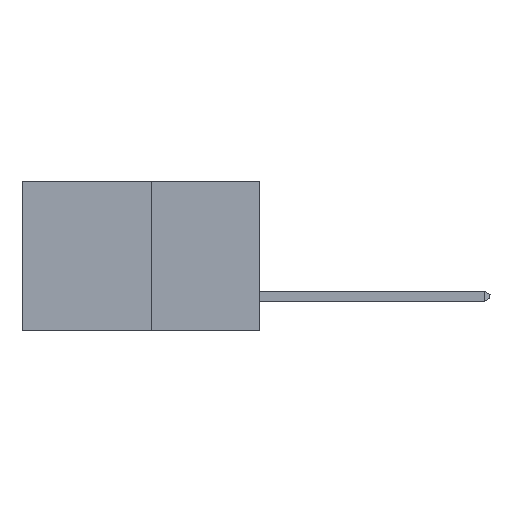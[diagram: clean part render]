
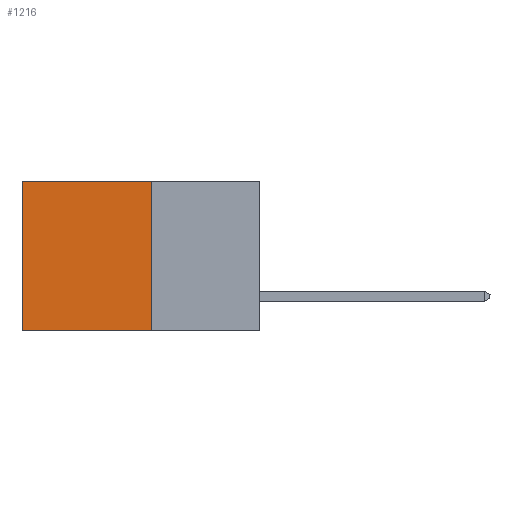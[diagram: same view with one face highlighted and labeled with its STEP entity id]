
A CAD part, left-side view. The second image highlights one B-rep face of the part: STEP entity #1216.
In plain terms, the highlighted planar face has unit normal (-1, 0, 0).
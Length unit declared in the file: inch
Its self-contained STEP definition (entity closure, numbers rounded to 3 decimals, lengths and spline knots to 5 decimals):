
#424 = CARTESIAN_POINT ( 'NONE',  ( 0.277, 0.27, -0.37 ) ) ;
#1216 = ADVANCED_FACE ( 'NONE', ( #18687 ), #19611, .F. ) ;
#1347 = EDGE_CURVE ( 'NONE', #5961, #11476, #3356, .T. ) ;
#3080 = VERTEX_POINT ( 'NONE', #15899 ) ;
#3356 = LINE ( 'NONE', #9914, #12105 ) ;
#3727 = VECTOR ( 'NONE', #16318, 39.37008 ) ;
#4156 = CARTESIAN_POINT ( 'NONE',  ( 0.277, 0.59, -0.37 ) ) ;
#4184 = CARTESIAN_POINT ( 'NONE',  ( 0.277, 0.27, 0. ) ) ;
#4206 = LINE ( 'NONE', #10052, #21698 ) ;
#4679 = LINE ( 'NONE', #14429, #18317 ) ;
#5961 = VERTEX_POINT ( 'NONE', #4184 ) ;
#8259 = ORIENTED_EDGE ( 'NONE', *, *, #1347, .F. ) ;
#9725 = DIRECTION ( 'NONE',  ( 0., 0., -1. ) ) ;
#9914 = CARTESIAN_POINT ( 'NONE',  ( 0.277, 0.27, -0.37 ) ) ;
#10052 = CARTESIAN_POINT ( 'NONE',  ( 0.277, 0.27, 0. ) ) ;
#11476 = VERTEX_POINT ( 'NONE', #21036 ) ;
#12105 = VECTOR ( 'NONE', #9725, 39.37008 ) ;
#13440 = EDGE_CURVE ( 'NONE', #3080, #17013, #21775, .T. ) ;
#14216 = EDGE_CURVE ( 'NONE', #5961, #3080, #4206, .T. ) ;
#14376 = AXIS2_PLACEMENT_3D ( 'NONE', #424, #21786, #15673 ) ;
#14429 = CARTESIAN_POINT ( 'NONE',  ( 0.277, 0.27, -0.37 ) ) ;
#14606 = CARTESIAN_POINT ( 'NONE',  ( 0.277, 0.59, -0.37 ) ) ;
#15673 = DIRECTION ( 'NONE',  ( 0., 0., -1. ) ) ;
#15899 = CARTESIAN_POINT ( 'NONE',  ( 0.277, 0.59, 0. ) ) ;
#16305 = EDGE_CURVE ( 'NONE', #11476, #17013, #4679, .T. ) ;
#16318 = DIRECTION ( 'NONE',  ( 0., 0., -1. ) ) ;
#17013 = VERTEX_POINT ( 'NONE', #4156 ) ;
#17161 = EDGE_LOOP ( 'NONE', ( #19147, #18636, #8259, #22031 ) ) ;
#18317 = VECTOR ( 'NONE', #20991, 39.37008 ) ;
#18636 = ORIENTED_EDGE ( 'NONE', *, *, #16305, .F. ) ;
#18687 = FACE_OUTER_BOUND ( 'NONE', #17161, .T. ) ;
#19147 = ORIENTED_EDGE ( 'NONE', *, *, #13440, .T. ) ;
#19611 = PLANE ( 'NONE',  #14376 ) ;
#20067 = DIRECTION ( 'NONE',  ( 0., 1., 0. ) ) ;
#20991 = DIRECTION ( 'NONE',  ( 0., 1., 0. ) ) ;
#21036 = CARTESIAN_POINT ( 'NONE',  ( 0.277, 0.27, -0.37 ) ) ;
#21698 = VECTOR ( 'NONE', #20067, 39.37008 ) ;
#21775 = LINE ( 'NONE', #14606, #3727 ) ;
#21786 = DIRECTION ( 'NONE',  ( 1., 0., 0. ) ) ;
#22031 = ORIENTED_EDGE ( 'NONE', *, *, #14216, .T. ) ;
